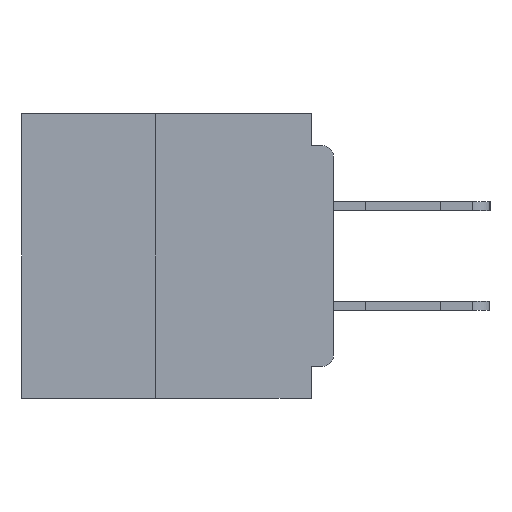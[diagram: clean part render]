
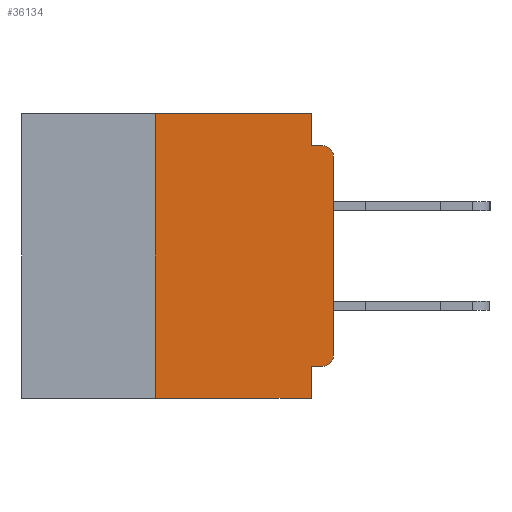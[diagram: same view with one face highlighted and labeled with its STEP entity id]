
A CAD part, left-side view. The second image highlights one B-rep face of the part: STEP entity #36134.
In plain terms, the highlighted planar face has unit normal (-1, 0, 0).
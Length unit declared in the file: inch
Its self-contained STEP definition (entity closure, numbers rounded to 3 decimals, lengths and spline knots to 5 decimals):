
#242 = CARTESIAN_POINT ( 'NONE',  ( 0., 0., -0.34 ) ) ;
#928 = DIRECTION ( 'NONE',  ( 0., -1., 0. ) ) ;
#1025 = VERTEX_POINT ( 'NONE', #9077 ) ;
#2000 = CARTESIAN_POINT ( 'NONE',  ( 0., 0.031, -0.045 ) ) ;
#2010 = ORIENTED_EDGE ( 'NONE', *, *, #42012, .F. ) ;
#2074 = LINE ( 'NONE', #45985, #21119 ) ;
#2239 = DIRECTION ( 'NONE',  ( 0., 0., -1. ) ) ;
#3708 = VERTEX_POINT ( 'NONE', #42840 ) ;
#4493 = CARTESIAN_POINT ( 'NONE',  ( 0., 0.25, 0. ) ) ;
#4570 = CARTESIAN_POINT ( 'NONE',  ( 0., 0.031, -0.4 ) ) ;
#5440 = EDGE_CURVE ( 'NONE', #22552, #1025, #36983, .T. ) ;
#6027 = DIRECTION ( 'NONE',  ( 0., 0., -1. ) ) ;
#6201 = PLANE ( 'NONE',  #15649 ) ;
#6798 = EDGE_CURVE ( 'NONE', #26222, #20578, #8074, .T. ) ;
#7461 = LINE ( 'NONE', #38716, #35174 ) ;
#7470 = CIRCLE ( 'NONE', #27946, 0.015 ) ;
#8034 = EDGE_CURVE ( 'NONE', #42361, #1025, #33897, .T. ) ;
#8048 = ORIENTED_EDGE ( 'NONE', *, *, #8034, .T. ) ;
#8074 = CIRCLE ( 'NONE', #18219, 0.015 ) ;
#9077 = CARTESIAN_POINT ( 'NONE',  ( 0., 0.031, -0.4 ) ) ;
#10047 = DIRECTION ( 'NONE',  ( 0., 0., -1. ) ) ;
#11812 = EDGE_LOOP ( 'NONE', ( #18664, #31063, #2010, #24590, #44391, #26966, #8048, #30508, #21682, #25227 ) ) ;
#11889 = CARTESIAN_POINT ( 'NONE',  ( 0., 0., -0.06 ) ) ;
#13110 = EDGE_CURVE ( 'NONE', #42361, #22419, #38809, .T. ) ;
#14003 = CARTESIAN_POINT ( 'NONE',  ( 0., 0., 0. ) ) ;
#14406 = EDGE_CURVE ( 'NONE', #34534, #3708, #7470, .T. ) ;
#15649 = AXIS2_PLACEMENT_3D ( 'NONE', #39912, #32617, #10047 ) ;
#16008 = EDGE_CURVE ( 'NONE', #20578, #34534, #47205, .T. ) ;
#17388 = CARTESIAN_POINT ( 'NONE',  ( 0., 0.015, -0.06 ) ) ;
#18183 = EDGE_CURVE ( 'NONE', #30224, #45492, #24027, .T. ) ;
#18219 = AXIS2_PLACEMENT_3D ( 'NONE', #47230, #25011, #2239 ) ;
#18664 = ORIENTED_EDGE ( 'NONE', *, *, #16008, .T. ) ;
#18854 = VECTOR ( 'NONE', #35227, 39.37008 ) ;
#18993 = LINE ( 'NONE', #20973, #26665 ) ;
#19690 = DIRECTION ( 'NONE',  ( 0., 0., -1. ) ) ;
#20578 = VERTEX_POINT ( 'NONE', #242 ) ;
#20973 = CARTESIAN_POINT ( 'NONE',  ( 0., 0., -0.355 ) ) ;
#21119 = VECTOR ( 'NONE', #928, 39.37008 ) ;
#21180 = DIRECTION ( 'NONE',  ( 0., 0., -1. ) ) ;
#21455 = CARTESIAN_POINT ( 'NONE',  ( 0., 0.437, -0.4 ) ) ;
#21682 = ORIENTED_EDGE ( 'NONE', *, *, #22005, .F. ) ;
#22005 = EDGE_CURVE ( 'NONE', #26222, #22552, #18993, .T. ) ;
#22419 = VERTEX_POINT ( 'NONE', #4493 ) ;
#22552 = VERTEX_POINT ( 'NONE', #42772 ) ;
#23427 = CARTESIAN_POINT ( 'NONE',  ( 0., 0.015, -0.355 ) ) ;
#24027 = LINE ( 'NONE', #28656, #34036 ) ;
#24590 = ORIENTED_EDGE ( 'NONE', *, *, #18183, .F. ) ;
#24762 = DIRECTION ( 'NONE',  ( 0., 1., 0. ) ) ;
#24940 = EDGE_CURVE ( 'NONE', #22419, #30224, #2074, .T. ) ;
#25011 = DIRECTION ( 'NONE',  ( -1., 0., 0. ) ) ;
#25227 = ORIENTED_EDGE ( 'NONE', *, *, #6798, .T. ) ;
#25881 = VECTOR ( 'NONE', #19690, 39.37008 ) ;
#26222 = VERTEX_POINT ( 'NONE', #23427 ) ;
#26665 = VECTOR ( 'NONE', #24762, 39.37008 ) ;
#26966 = ORIENTED_EDGE ( 'NONE', *, *, #13110, .F. ) ;
#27500 = VECTOR ( 'NONE', #40239, 39.37008 ) ;
#27946 = AXIS2_PLACEMENT_3D ( 'NONE', #17388, #43511, #21180 ) ;
#28656 = CARTESIAN_POINT ( 'NONE',  ( 0., 0.031, 0. ) ) ;
#29567 = CARTESIAN_POINT ( 'NONE',  ( 0., 0.25, -0.4 ) ) ;
#30224 = VERTEX_POINT ( 'NONE', #32922 ) ;
#30508 = ORIENTED_EDGE ( 'NONE', *, *, #5440, .F. ) ;
#31063 = ORIENTED_EDGE ( 'NONE', *, *, #14406, .T. ) ;
#31396 = DIRECTION ( 'NONE',  ( 0., -1., 0. ) ) ;
#31480 = CARTESIAN_POINT ( 'NONE',  ( 0., 0.25, -0.4 ) ) ;
#31567 = VECTOR ( 'NONE', #47300, 39.37008 ) ;
#32617 = DIRECTION ( 'NONE',  ( 1., 0., 0. ) ) ;
#32922 = CARTESIAN_POINT ( 'NONE',  ( 0., 0.031, 0. ) ) ;
#33897 = LINE ( 'NONE', #21455, #31567 ) ;
#34036 = VECTOR ( 'NONE', #6027, 39.37008 ) ;
#34534 = VERTEX_POINT ( 'NONE', #11889 ) ;
#35174 = VECTOR ( 'NONE', #31396, 39.37008 ) ;
#35227 = DIRECTION ( 'NONE',  ( 0., 0., 1. ) ) ;
#36134 = ADVANCED_FACE ( 'NONE', ( #39611 ), #6201, .F. ) ;
#36983 = LINE ( 'NONE', #4570, #25881 ) ;
#38716 = CARTESIAN_POINT ( 'NONE',  ( 0., 0., -0.045 ) ) ;
#38809 = LINE ( 'NONE', #31480, #18854 ) ;
#39611 = FACE_OUTER_BOUND ( 'NONE', #11812, .T. ) ;
#39912 = CARTESIAN_POINT ( 'NONE',  ( 0., 0.437, 0. ) ) ;
#40239 = DIRECTION ( 'NONE',  ( 0., 0., 1. ) ) ;
#42012 = EDGE_CURVE ( 'NONE', #45492, #3708, #7461, .T. ) ;
#42361 = VERTEX_POINT ( 'NONE', #29567 ) ;
#42772 = CARTESIAN_POINT ( 'NONE',  ( 0., 0.031, -0.355 ) ) ;
#42840 = CARTESIAN_POINT ( 'NONE',  ( 0., 0.015, -0.045 ) ) ;
#43511 = DIRECTION ( 'NONE',  ( -1., 0., 0. ) ) ;
#44391 = ORIENTED_EDGE ( 'NONE', *, *, #24940, .F. ) ;
#45492 = VERTEX_POINT ( 'NONE', #2000 ) ;
#45985 = CARTESIAN_POINT ( 'NONE',  ( 0., 0.437, 0. ) ) ;
#47205 = LINE ( 'NONE', #14003, #27500 ) ;
#47230 = CARTESIAN_POINT ( 'NONE',  ( 0., 0.015, -0.34 ) ) ;
#47300 = DIRECTION ( 'NONE',  ( 0., -1., 0. ) ) ;
